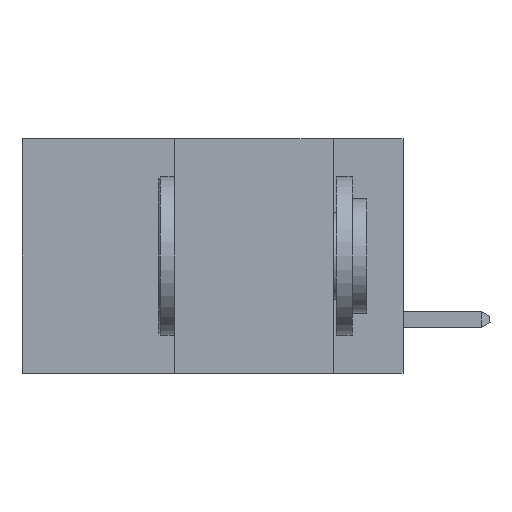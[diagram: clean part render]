
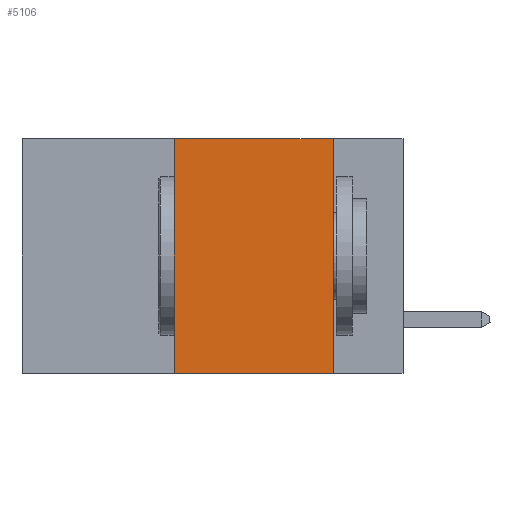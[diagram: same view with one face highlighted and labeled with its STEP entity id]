
A CAD part, left-side view. The second image highlights one B-rep face of the part: STEP entity #5106.
In plain terms, the highlighted planar face has unit normal (-1, 0, 0).
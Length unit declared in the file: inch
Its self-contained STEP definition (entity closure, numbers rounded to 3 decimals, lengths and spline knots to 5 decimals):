
#523 = VECTOR ( 'NONE', #15055, 39.37008 ) ;
#692 = CARTESIAN_POINT ( 'NONE',  ( 0., 0.11, 0. ) ) ;
#2631 = VERTEX_POINT ( 'NONE', #2893 ) ;
#2893 = CARTESIAN_POINT ( 'NONE',  ( 0., 0.36, 0. ) ) ;
#3172 = VERTEX_POINT ( 'NONE', #17563 ) ;
#3455 = CARTESIAN_POINT ( 'NONE',  ( 0., 0.6, -0.37 ) ) ;
#4635 = EDGE_CURVE ( 'NONE', #2631, #17550, #17342, .T. ) ;
#4880 = DIRECTION ( 'NONE',  ( 0., -1., 0. ) ) ;
#5106 = ADVANCED_FACE ( 'NONE', ( #17324 ), #7767, .F. ) ;
#5116 = DIRECTION ( 'NONE',  ( 0., 0., -1. ) ) ;
#6709 = VECTOR ( 'NONE', #16207, 39.37008 ) ;
#6792 = CARTESIAN_POINT ( 'NONE',  ( 0., 0.11, -0.37 ) ) ;
#7461 = EDGE_CURVE ( 'NONE', #3172, #2631, #14369, .T. ) ;
#7499 = LINE ( 'NONE', #11080, #523 ) ;
#7530 = VERTEX_POINT ( 'NONE', #6792 ) ;
#7713 = ORIENTED_EDGE ( 'NONE', *, *, #15508, .F. ) ;
#7767 = PLANE ( 'NONE',  #10071 ) ;
#7984 = ORIENTED_EDGE ( 'NONE', *, *, #4635, .F. ) ;
#8158 = ORIENTED_EDGE ( 'NONE', *, *, #7461, .F. ) ;
#10071 = AXIS2_PLACEMENT_3D ( 'NONE', #11785, #13153, #5116 ) ;
#10101 = VECTOR ( 'NONE', #4880, 39.37008 ) ;
#10183 = ORIENTED_EDGE ( 'NONE', *, *, #11372, .T. ) ;
#10639 = CARTESIAN_POINT ( 'NONE',  ( 0., 0.36, 0. ) ) ;
#10774 = VECTOR ( 'NONE', #14697, 39.37008 ) ;
#11080 = CARTESIAN_POINT ( 'NONE',  ( 0., 0.11, 0. ) ) ;
#11372 = EDGE_CURVE ( 'NONE', #3172, #7530, #14116, .T. ) ;
#11785 = CARTESIAN_POINT ( 'NONE',  ( 0., 0.6, 0. ) ) ;
#13153 = DIRECTION ( 'NONE',  ( 1., 0., 0. ) ) ;
#13426 = EDGE_LOOP ( 'NONE', ( #7713, #7984, #8158, #10183 ) ) ;
#14116 = LINE ( 'NONE', #3455, #10101 ) ;
#14369 = LINE ( 'NONE', #10639, #10774 ) ;
#14697 = DIRECTION ( 'NONE',  ( 0., 0., 1. ) ) ;
#14917 = CARTESIAN_POINT ( 'NONE',  ( 0., 0.6, 0. ) ) ;
#15055 = DIRECTION ( 'NONE',  ( 0., 0., -1. ) ) ;
#15508 = EDGE_CURVE ( 'NONE', #17550, #7530, #7499, .T. ) ;
#16207 = DIRECTION ( 'NONE',  ( 0., -1., 0. ) ) ;
#17324 = FACE_OUTER_BOUND ( 'NONE', #13426, .T. ) ;
#17342 = LINE ( 'NONE', #14917, #6709 ) ;
#17550 = VERTEX_POINT ( 'NONE', #692 ) ;
#17563 = CARTESIAN_POINT ( 'NONE',  ( 0., 0.36, -0.37 ) ) ;
